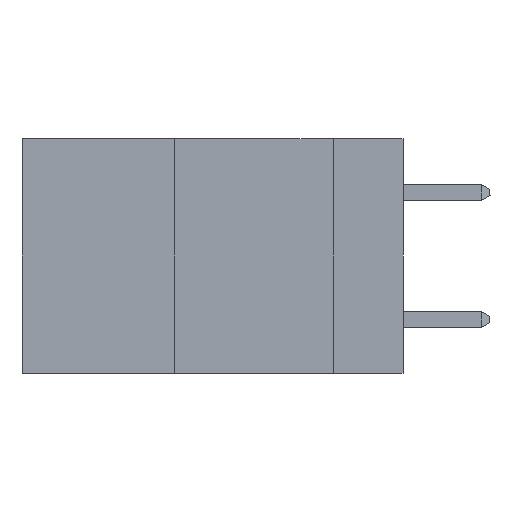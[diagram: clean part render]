
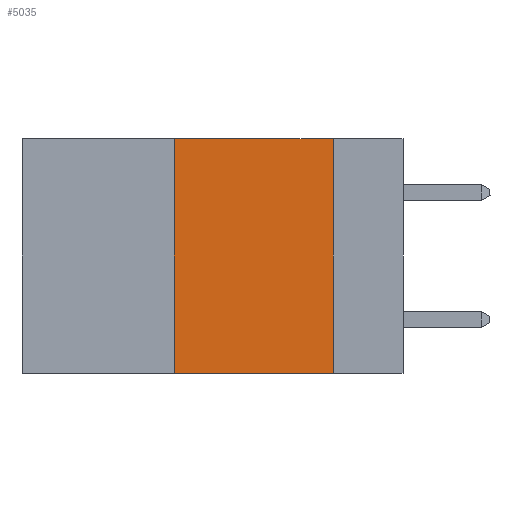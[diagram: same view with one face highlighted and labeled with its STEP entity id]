
A CAD part, left-side view. The second image highlights one B-rep face of the part: STEP entity #5035.
In plain terms, the highlighted planar face has unit normal (-1, 0, 0).
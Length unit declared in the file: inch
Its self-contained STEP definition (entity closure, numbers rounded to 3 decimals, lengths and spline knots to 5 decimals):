
#476 = LINE ( 'NONE', #12771, #15286 ) ;
#731 = VERTEX_POINT ( 'NONE', #21208 ) ;
#849 = ORIENTED_EDGE ( 'NONE', *, *, #21213, .F. ) ;
#2011 = CARTESIAN_POINT ( 'NONE',  ( 0., 0.11, 0. ) ) ;
#2043 = CARTESIAN_POINT ( 'NONE',  ( 0., 0.6, 0. ) ) ;
#2054 = VECTOR ( 'NONE', #2845, 39.37008 ) ;
#2569 = PLANE ( 'NONE',  #14894 ) ;
#2588 = CARTESIAN_POINT ( 'NONE',  ( 0., 0.6, -0.37 ) ) ;
#2596 = VERTEX_POINT ( 'NONE', #2011 ) ;
#2845 = DIRECTION ( 'NONE',  ( 0., -1., 0. ) ) ;
#3398 = DIRECTION ( 'NONE',  ( 0., 0., -1. ) ) ;
#4164 = DIRECTION ( 'NONE',  ( 1., 0., 0. ) ) ;
#4256 = ORIENTED_EDGE ( 'NONE', *, *, #24104, .F. ) ;
#4501 = LINE ( 'NONE', #10656, #9649 ) ;
#5035 = ADVANCED_FACE ( 'NONE', ( #22478 ), #2569, .F. ) ;
#7071 = CARTESIAN_POINT ( 'NONE',  ( 0., 0.36, -0.37 ) ) ;
#7290 = DIRECTION ( 'NONE',  ( 0., 0., 1. ) ) ;
#7398 = LINE ( 'NONE', #20088, #26325 ) ;
#7460 = ORIENTED_EDGE ( 'NONE', *, *, #20536, .F. ) ;
#9649 = VECTOR ( 'NONE', #7290, 39.37008 ) ;
#10656 = CARTESIAN_POINT ( 'NONE',  ( 0., 0.36, 0. ) ) ;
#11672 = CARTESIAN_POINT ( 'NONE',  ( 0., 0.36, 0. ) ) ;
#12184 = VERTEX_POINT ( 'NONE', #11672 ) ;
#12771 = CARTESIAN_POINT ( 'NONE',  ( 0., 0.6, 0. ) ) ;
#13558 = ORIENTED_EDGE ( 'NONE', *, *, #22752, .T. ) ;
#14894 = AXIS2_PLACEMENT_3D ( 'NONE', #2043, #4164, #22738 ) ;
#15286 = VECTOR ( 'NONE', #20921, 39.37008 ) ;
#15408 = LINE ( 'NONE', #2588, #2054 ) ;
#20088 = CARTESIAN_POINT ( 'NONE',  ( 0., 0.11, 0. ) ) ;
#20536 = EDGE_CURVE ( 'NONE', #23279, #12184, #4501, .T. ) ;
#20921 = DIRECTION ( 'NONE',  ( 0., -1., 0. ) ) ;
#21208 = CARTESIAN_POINT ( 'NONE',  ( 0., 0.11, -0.37 ) ) ;
#21213 = EDGE_CURVE ( 'NONE', #2596, #731, #7398, .T. ) ;
#22478 = FACE_OUTER_BOUND ( 'NONE', #23737, .T. ) ;
#22738 = DIRECTION ( 'NONE',  ( 0., 0., -1. ) ) ;
#22752 = EDGE_CURVE ( 'NONE', #23279, #731, #15408, .T. ) ;
#23279 = VERTEX_POINT ( 'NONE', #7071 ) ;
#23737 = EDGE_LOOP ( 'NONE', ( #849, #4256, #7460, #13558 ) ) ;
#24104 = EDGE_CURVE ( 'NONE', #12184, #2596, #476, .T. ) ;
#26325 = VECTOR ( 'NONE', #3398, 39.37008 ) ;
